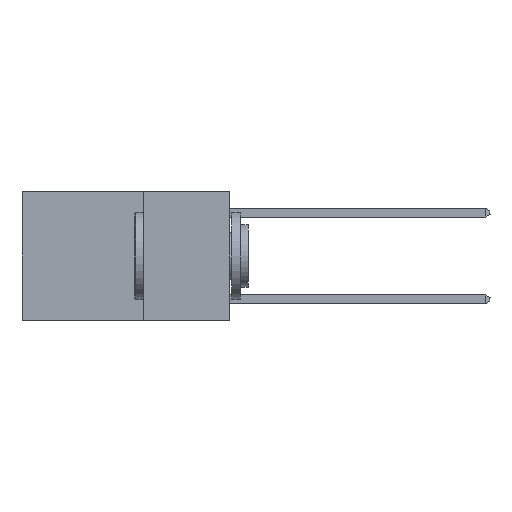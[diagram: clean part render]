
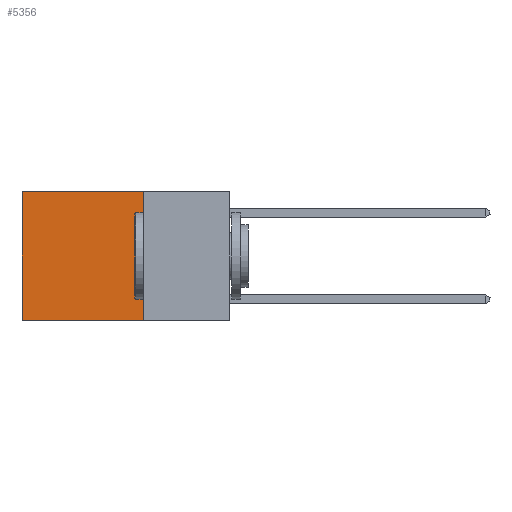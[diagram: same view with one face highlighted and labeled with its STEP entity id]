
A CAD part, left-side view. The second image highlights one B-rep face of the part: STEP entity #5356.
In plain terms, the highlighted planar face has unit normal (-1, 0, 0).
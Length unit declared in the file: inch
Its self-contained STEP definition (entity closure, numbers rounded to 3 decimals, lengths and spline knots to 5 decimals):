
#340 = ORIENTED_EDGE ( 'NONE', *, *, #17402, .F. ) ;
#1004 = CARTESIAN_POINT ( 'NONE',  ( 0.2625, 0.25, 0. ) ) ;
#1997 = ORIENTED_EDGE ( 'NONE', *, *, #16954, .T. ) ;
#2360 = VERTEX_POINT ( 'NONE', #18704 ) ;
#2420 = CARTESIAN_POINT ( 'NONE',  ( 0.2625, 0.6, 0. ) ) ;
#2585 = CARTESIAN_POINT ( 'NONE',  ( 0.2625, 0.25, 0. ) ) ;
#4400 = LINE ( 'NONE', #2585, #15395 ) ;
#5356 = ADVANCED_FACE ( 'NONE', ( #6402 ), #14130, .F. ) ;
#6259 = LINE ( 'NONE', #13632, #14813 ) ;
#6402 = FACE_OUTER_BOUND ( 'NONE', #22978, .T. ) ;
#7210 = AXIS2_PLACEMENT_3D ( 'NONE', #15937, #21027, #17619 ) ;
#7549 = VERTEX_POINT ( 'NONE', #13673 ) ;
#8266 = ORIENTED_EDGE ( 'NONE', *, *, #8712, .T. ) ;
#8712 = EDGE_CURVE ( 'NONE', #23456, #20686, #4400, .T. ) ;
#9609 = DIRECTION ( 'NONE',  ( 0., 1., 0. ) ) ;
#9743 = DIRECTION ( 'NONE',  ( 0., 0., -1. ) ) ;
#11560 = CARTESIAN_POINT ( 'NONE',  ( 0.2625, 0.25, 0. ) ) ;
#11703 = ORIENTED_EDGE ( 'NONE', *, *, #19998, .F. ) ;
#11715 = VECTOR ( 'NONE', #15440, 39.37008 ) ;
#13592 = VECTOR ( 'NONE', #9743, 39.37008 ) ;
#13632 = CARTESIAN_POINT ( 'NONE',  ( 0.2625, 0.25, -0.37 ) ) ;
#13673 = CARTESIAN_POINT ( 'NONE',  ( 0.2625, 0.6, -0.37 ) ) ;
#14130 = PLANE ( 'NONE',  #7210 ) ;
#14813 = VECTOR ( 'NONE', #21006, 39.37008 ) ;
#15395 = VECTOR ( 'NONE', #9609, 39.37008 ) ;
#15440 = DIRECTION ( 'NONE',  ( 0., 0., -1. ) ) ;
#15937 = CARTESIAN_POINT ( 'NONE',  ( 0.2625, 0.25, 0. ) ) ;
#16954 = EDGE_CURVE ( 'NONE', #20686, #7549, #21011, .T. ) ;
#17402 = EDGE_CURVE ( 'NONE', #23456, #2360, #19381, .T. ) ;
#17619 = DIRECTION ( 'NONE',  ( 0., 0., -1. ) ) ;
#18704 = CARTESIAN_POINT ( 'NONE',  ( 0.2625, 0.25, -0.37 ) ) ;
#19381 = LINE ( 'NONE', #11560, #13592 ) ;
#19998 = EDGE_CURVE ( 'NONE', #2360, #7549, #6259, .T. ) ;
#20686 = VERTEX_POINT ( 'NONE', #2420 ) ;
#21006 = DIRECTION ( 'NONE',  ( 0., 1., 0. ) ) ;
#21011 = LINE ( 'NONE', #21132, #11715 ) ;
#21027 = DIRECTION ( 'NONE',  ( 1., 0., 0. ) ) ;
#21132 = CARTESIAN_POINT ( 'NONE',  ( 0.2625, 0.6, 0. ) ) ;
#22978 = EDGE_LOOP ( 'NONE', ( #1997, #11703, #340, #8266 ) ) ;
#23456 = VERTEX_POINT ( 'NONE', #1004 ) ;
